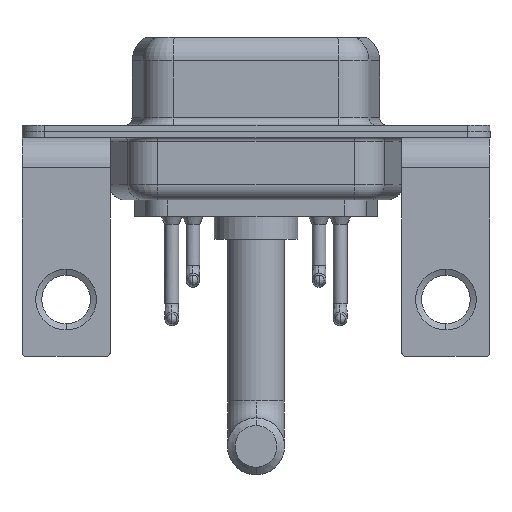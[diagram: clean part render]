
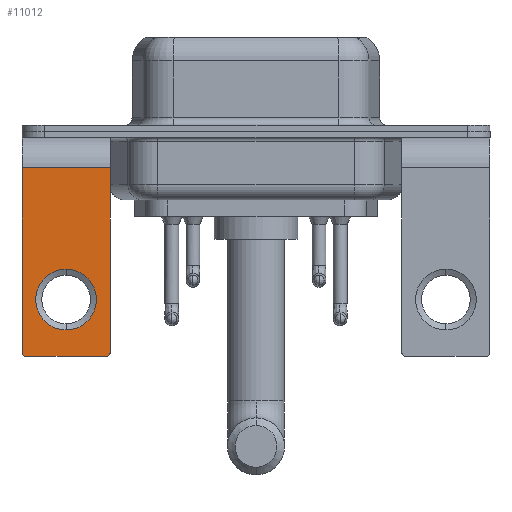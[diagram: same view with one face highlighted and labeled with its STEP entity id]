
A CAD part, front view. The second image highlights one B-rep face of the part: STEP entity #11012.
In plain terms, the highlighted planar face has unit normal (0, -1, 0).
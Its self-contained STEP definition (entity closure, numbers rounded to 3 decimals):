
#116 = VERTEX_POINT ( 'NONE', #12338 ) ;
#455 = VERTEX_POINT ( 'NONE', #5624 ) ;
#838 = CIRCLE ( 'NONE', #5005, 0.25 ) ;
#1150 = ORIENTED_EDGE ( 'NONE', *, *, #4376, .T. ) ;
#1542 = CARTESIAN_POINT ( 'NONE',  ( 2.9, -6.25, -14.8 ) ) ;
#2537 = ORIENTED_EDGE ( 'NONE', *, *, #9654, .F. ) ;
#2630 = CARTESIAN_POINT ( 'NONE',  ( -2.65, -6.25, -14.8 ) ) ;
#2652 = CARTESIAN_POINT ( 'NONE',  ( 2.9, -6.25, -14.55 ) ) ;
#2770 = ORIENTED_EDGE ( 'NONE', *, *, #4594, .F. ) ;
#3118 = VECTOR ( 'NONE', #14879, 1000. ) ;
#3304 = DIRECTION ( 'NONE',  ( 0., 1., 0. ) ) ;
#3576 = DIRECTION ( 'NONE',  ( 0., 1., 0. ) ) ;
#3593 = DIRECTION ( 'NONE',  ( 0., 0., -1. ) ) ;
#3646 = CARTESIAN_POINT ( 'NONE',  ( -2.65, -6.25, -14.55 ) ) ;
#4002 = LINE ( 'NONE', #12073, #14746 ) ;
#4169 = AXIS2_PLACEMENT_3D ( 'NONE', #16699, #14030, #4907 ) ;
#4369 = EDGE_CURVE ( 'NONE', #116, #15807, #10834, .T. ) ;
#4376 = EDGE_CURVE ( 'NONE', #6420, #15000, #6883, .T. ) ;
#4380 = CARTESIAN_POINT ( 'NONE',  ( 2.9, -6.25, -2.4 ) ) ;
#4594 = EDGE_CURVE ( 'NONE', #6420, #15807, #4002, .T. ) ;
#4714 = LINE ( 'NONE', #14098, #14016 ) ;
#4789 = EDGE_CURVE ( 'NONE', #455, #8346, #6485, .T. ) ;
#4790 = PLANE ( 'NONE',  #7371 ) ;
#4907 = DIRECTION ( 'NONE',  ( 0., 0., 1. ) ) ;
#5000 = ORIENTED_EDGE ( 'NONE', *, *, #7637, .T. ) ;
#5005 = AXIS2_PLACEMENT_3D ( 'NONE', #3646, #14315, #14227 ) ;
#5523 = DIRECTION ( 'NONE',  ( -1., 0., 0. ) ) ;
#5624 = CARTESIAN_POINT ( 'NONE',  ( 0., -6.25, -13.07 ) ) ;
#6317 = CARTESIAN_POINT ( 'NONE',  ( 0., -6.25, -9.07 ) ) ;
#6420 = VERTEX_POINT ( 'NONE', #6430 ) ;
#6430 = CARTESIAN_POINT ( 'NONE',  ( 2.9, -6.25, -2.4 ) ) ;
#6485 = CIRCLE ( 'NONE', #8141, 2. ) ;
#6883 = LINE ( 'NONE', #4380, #3118 ) ;
#7205 = EDGE_CURVE ( 'NONE', #8346, #455, #15442, .T. ) ;
#7371 = AXIS2_PLACEMENT_3D ( 'NONE', #12694, #3576, #11395 ) ;
#7523 = FACE_OUTER_BOUND ( 'NONE', #16509, .T. ) ;
#7637 = EDGE_CURVE ( 'NONE', #15000, #11703, #4714, .T. ) ;
#7852 = ORIENTED_EDGE ( 'NONE', *, *, #4789, .T. ) ;
#8141 = AXIS2_PLACEMENT_3D ( 'NONE', #10964, #3304, #10885 ) ;
#8346 = VERTEX_POINT ( 'NONE', #6317 ) ;
#8520 = LINE ( 'NONE', #1542, #12034 ) ;
#9654 = EDGE_CURVE ( 'NONE', #116, #14860, #8520, .T. ) ;
#10834 = CIRCLE ( 'NONE', #13342, 0.25 ) ;
#10885 = DIRECTION ( 'NONE',  ( 0., 0., 1. ) ) ;
#10964 = CARTESIAN_POINT ( 'NONE',  ( 0., -6.25, -11.07 ) ) ;
#11012 = ADVANCED_FACE ( 'NONE', ( #15357, #7523 ), #4790, .F. ) ;
#11395 = DIRECTION ( 'NONE',  ( 0., 0., 1. ) ) ;
#11694 = EDGE_LOOP ( 'NONE', ( #7852, #16370 ) ) ;
#11703 = VERTEX_POINT ( 'NONE', #16142 ) ;
#12034 = VECTOR ( 'NONE', #5523, 1000. ) ;
#12073 = CARTESIAN_POINT ( 'NONE',  ( 2.9, -6.25, -2.4 ) ) ;
#12094 = CARTESIAN_POINT ( 'NONE',  ( -2.9, -6.25, -2.4 ) ) ;
#12338 = CARTESIAN_POINT ( 'NONE',  ( 2.65, -6.25, -14.8 ) ) ;
#12694 = CARTESIAN_POINT ( 'NONE',  ( 2.9, -6.25, -2.4 ) ) ;
#13342 = AXIS2_PLACEMENT_3D ( 'NONE', #14974, #13516, #16168 ) ;
#13516 = DIRECTION ( 'NONE',  ( 0., -1., 0. ) ) ;
#13918 = EDGE_CURVE ( 'NONE', #11703, #14860, #838, .T. ) ;
#14002 = ORIENTED_EDGE ( 'NONE', *, *, #13918, .T. ) ;
#14016 = VECTOR ( 'NONE', #3593, 1000. ) ;
#14030 = DIRECTION ( 'NONE',  ( 0., 1., 0. ) ) ;
#14098 = CARTESIAN_POINT ( 'NONE',  ( -2.9, -6.25, -2.4 ) ) ;
#14227 = DIRECTION ( 'NONE',  ( 0., 0., 1. ) ) ;
#14315 = DIRECTION ( 'NONE',  ( 0., -1., 0. ) ) ;
#14387 = ORIENTED_EDGE ( 'NONE', *, *, #4369, .T. ) ;
#14588 = DIRECTION ( 'NONE',  ( 0., 0., -1. ) ) ;
#14746 = VECTOR ( 'NONE', #14588, 1000. ) ;
#14860 = VERTEX_POINT ( 'NONE', #2630 ) ;
#14879 = DIRECTION ( 'NONE',  ( -1., 0., 0. ) ) ;
#14974 = CARTESIAN_POINT ( 'NONE',  ( 2.65, -6.25, -14.55 ) ) ;
#15000 = VERTEX_POINT ( 'NONE', #12094 ) ;
#15357 = FACE_BOUND ( 'NONE', #11694, .T. ) ;
#15442 = CIRCLE ( 'NONE', #4169, 2. ) ;
#15807 = VERTEX_POINT ( 'NONE', #2652 ) ;
#16142 = CARTESIAN_POINT ( 'NONE',  ( -2.9, -6.25, -14.55 ) ) ;
#16168 = DIRECTION ( 'NONE',  ( 0., 0., 1. ) ) ;
#16370 = ORIENTED_EDGE ( 'NONE', *, *, #7205, .T. ) ;
#16509 = EDGE_LOOP ( 'NONE', ( #5000, #14002, #2537, #14387, #2770, #1150 ) ) ;
#16699 = CARTESIAN_POINT ( 'NONE',  ( 0., -6.25, -11.07 ) ) ;
